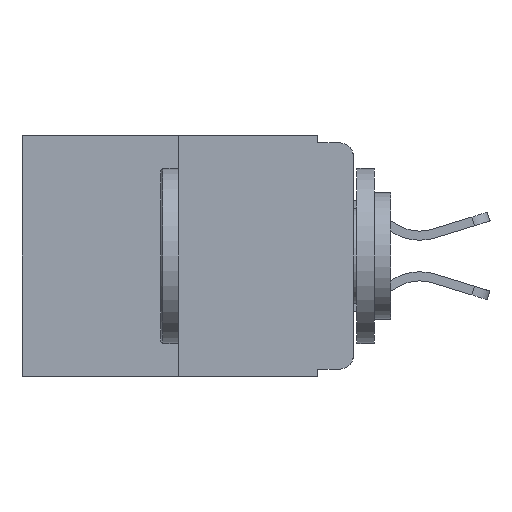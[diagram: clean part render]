
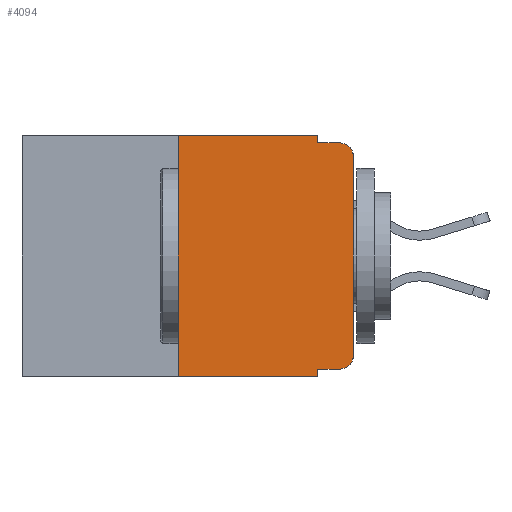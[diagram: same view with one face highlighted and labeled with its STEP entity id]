
A CAD part, left-side view. The second image highlights one B-rep face of the part: STEP entity #4094.
In plain terms, the highlighted planar face has unit normal (-1, 0, 0).
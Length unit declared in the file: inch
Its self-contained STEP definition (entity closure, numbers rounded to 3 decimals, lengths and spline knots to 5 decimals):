
#81 = DIRECTION ( 'NONE',  ( -1., 0., 0. ) ) ;
#543 = EDGE_LOOP ( 'NONE', ( #858, #8095, #13530, #15874, #21695, #19057, #20716, #12420, #9401, #10374 ) ) ;
#668 = VECTOR ( 'NONE', #12037, 39.37008 ) ;
#858 = ORIENTED_EDGE ( 'NONE', *, *, #15361, .T. ) ;
#1008 = VECTOR ( 'NONE', #18608, 39.37008 ) ;
#1209 = AXIS2_PLACEMENT_3D ( 'NONE', #14083, #81, #12529 ) ;
#1401 = FACE_OUTER_BOUND ( 'NONE', #543, .T. ) ;
#1491 = AXIS2_PLACEMENT_3D ( 'NONE', #22550, #20767, #6577 ) ;
#4094 = ADVANCED_FACE ( 'NONE', ( #1401 ), #15504, .F. ) ;
#4243 = CARTESIAN_POINT ( 'NONE',  ( 0., 0.02, -0.01 ) ) ;
#4409 = CARTESIAN_POINT ( 'NONE',  ( 0., 0., 0. ) ) ;
#4447 = CARTESIAN_POINT ( 'NONE',  ( 0., 0.051, 0. ) ) ;
#4979 = CARTESIAN_POINT ( 'NONE',  ( 0., 0.02, -0.333 ) ) ;
#5120 = VERTEX_POINT ( 'NONE', #19939 ) ;
#5385 = DIRECTION ( 'NONE',  ( 0., 0., -1. ) ) ;
#5441 = EDGE_CURVE ( 'NONE', #5447, #15652, #17742, .T. ) ;
#5447 = VERTEX_POINT ( 'NONE', #11925 ) ;
#5529 = VECTOR ( 'NONE', #20720, 39.37008 ) ;
#5581 = DIRECTION ( 'NONE',  ( 0., -1., 0. ) ) ;
#6431 = CARTESIAN_POINT ( 'NONE',  ( 0., 0.051, -0.01 ) ) ;
#6577 = DIRECTION ( 'NONE',  ( 0., 0., -1. ) ) ;
#6919 = CIRCLE ( 'NONE', #7912, 0.02 ) ;
#7101 = CARTESIAN_POINT ( 'NONE',  ( 0., 0.25, -0.343 ) ) ;
#7382 = VERTEX_POINT ( 'NONE', #21426 ) ;
#7680 = VECTOR ( 'NONE', #18470, 39.37008 ) ;
#7902 = LINE ( 'NONE', #16080, #8736 ) ;
#7912 = AXIS2_PLACEMENT_3D ( 'NONE', #21460, #10612, #5385 ) ;
#8095 = ORIENTED_EDGE ( 'NONE', *, *, #20577, .T. ) ;
#8319 = CARTESIAN_POINT ( 'NONE',  ( 0., 0.051, 0. ) ) ;
#8533 = VERTEX_POINT ( 'NONE', #22312 ) ;
#8736 = VECTOR ( 'NONE', #5581, 39.37008 ) ;
#8846 = VERTEX_POINT ( 'NONE', #4243 ) ;
#9052 = VECTOR ( 'NONE', #15333, 39.37008 ) ;
#9119 = LINE ( 'NONE', #22367, #1008 ) ;
#9401 = ORIENTED_EDGE ( 'NONE', *, *, #17177, .T. ) ;
#9444 = LINE ( 'NONE', #4409, #5529 ) ;
#9676 = CARTESIAN_POINT ( 'NONE',  ( 0., 0.473, -0.343 ) ) ;
#10145 = CARTESIAN_POINT ( 'NONE',  ( 0., 0.25, 0. ) ) ;
#10298 = VECTOR ( 'NONE', #11356, 39.37008 ) ;
#10374 = ORIENTED_EDGE ( 'NONE', *, *, #15080, .T. ) ;
#10612 = DIRECTION ( 'NONE',  ( -1., 0., 0. ) ) ;
#10809 = EDGE_CURVE ( 'NONE', #21298, #22487, #16084, .T. ) ;
#11356 = DIRECTION ( 'NONE',  ( 0., -1., 0. ) ) ;
#11429 = EDGE_CURVE ( 'NONE', #21298, #8533, #14671, .T. ) ;
#11925 = CARTESIAN_POINT ( 'NONE',  ( 0., 0.051, 0. ) ) ;
#12037 = DIRECTION ( 'NONE',  ( 0., 0., 1. ) ) ;
#12238 = EDGE_CURVE ( 'NONE', #5120, #22487, #18301, .T. ) ;
#12420 = ORIENTED_EDGE ( 'NONE', *, *, #12238, .F. ) ;
#12529 = DIRECTION ( 'NONE',  ( 0., 0., -1. ) ) ;
#13016 = CARTESIAN_POINT ( 'NONE',  ( 0., 0.051, -0.343 ) ) ;
#13092 = CIRCLE ( 'NONE', #1209, 0.02 ) ;
#13530 = ORIENTED_EDGE ( 'NONE', *, *, #19658, .F. ) ;
#13778 = DIRECTION ( 'NONE',  ( 0., 0., -1. ) ) ;
#13924 = VERTEX_POINT ( 'NONE', #4979 ) ;
#14083 = CARTESIAN_POINT ( 'NONE',  ( 0., 0.02, -0.313 ) ) ;
#14671 = LINE ( 'NONE', #10145, #668 ) ;
#15080 = EDGE_CURVE ( 'NONE', #13924, #18917, #13092, .T. ) ;
#15333 = DIRECTION ( 'NONE',  ( 0., 0., -1. ) ) ;
#15361 = EDGE_CURVE ( 'NONE', #18917, #7382, #9444, .T. ) ;
#15504 = PLANE ( 'NONE',  #1491 ) ;
#15652 = VERTEX_POINT ( 'NONE', #6431 ) ;
#15874 = ORIENTED_EDGE ( 'NONE', *, *, #5441, .F. ) ;
#16080 = CARTESIAN_POINT ( 'NONE',  ( 0., 0.051, -0.333 ) ) ;
#16084 = LINE ( 'NONE', #9676, #7680 ) ;
#16686 = EDGE_CURVE ( 'NONE', #8533, #5447, #9119, .T. ) ;
#16760 = CARTESIAN_POINT ( 'NONE',  ( 0., 0.051, -0.01 ) ) ;
#17177 = EDGE_CURVE ( 'NONE', #5120, #13924, #7902, .T. ) ;
#17307 = LINE ( 'NONE', #16760, #10298 ) ;
#17742 = LINE ( 'NONE', #8319, #19985 ) ;
#18301 = LINE ( 'NONE', #4447, #9052 ) ;
#18470 = DIRECTION ( 'NONE',  ( 0., -1., 0. ) ) ;
#18608 = DIRECTION ( 'NONE',  ( 0., -1., 0. ) ) ;
#18917 = VERTEX_POINT ( 'NONE', #21664 ) ;
#19057 = ORIENTED_EDGE ( 'NONE', *, *, #11429, .F. ) ;
#19658 = EDGE_CURVE ( 'NONE', #15652, #8846, #17307, .T. ) ;
#19939 = CARTESIAN_POINT ( 'NONE',  ( 0., 0.051, -0.333 ) ) ;
#19985 = VECTOR ( 'NONE', #13778, 39.37008 ) ;
#20577 = EDGE_CURVE ( 'NONE', #7382, #8846, #6919, .T. ) ;
#20716 = ORIENTED_EDGE ( 'NONE', *, *, #10809, .T. ) ;
#20720 = DIRECTION ( 'NONE',  ( 0., 0., 1. ) ) ;
#20767 = DIRECTION ( 'NONE',  ( 1., 0., 0. ) ) ;
#21298 = VERTEX_POINT ( 'NONE', #7101 ) ;
#21426 = CARTESIAN_POINT ( 'NONE',  ( 0., 0., -0.03 ) ) ;
#21460 = CARTESIAN_POINT ( 'NONE',  ( 0., 0.02, -0.03 ) ) ;
#21664 = CARTESIAN_POINT ( 'NONE',  ( 0., 0., -0.313 ) ) ;
#21695 = ORIENTED_EDGE ( 'NONE', *, *, #16686, .F. ) ;
#22312 = CARTESIAN_POINT ( 'NONE',  ( 0., 0.25, 0. ) ) ;
#22367 = CARTESIAN_POINT ( 'NONE',  ( 0., 0.473, 0. ) ) ;
#22487 = VERTEX_POINT ( 'NONE', #13016 ) ;
#22550 = CARTESIAN_POINT ( 'NONE',  ( 0., 0.473, 0. ) ) ;
